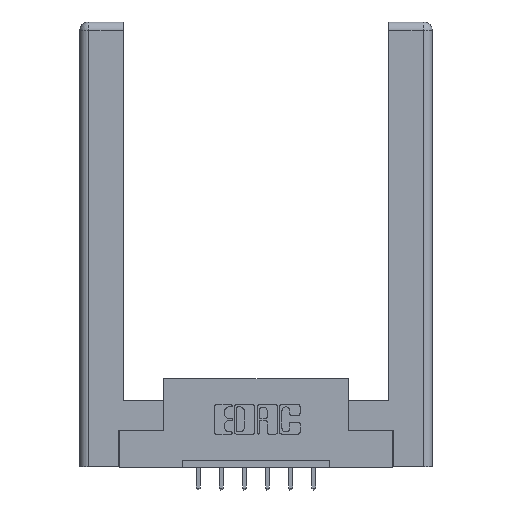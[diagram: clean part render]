
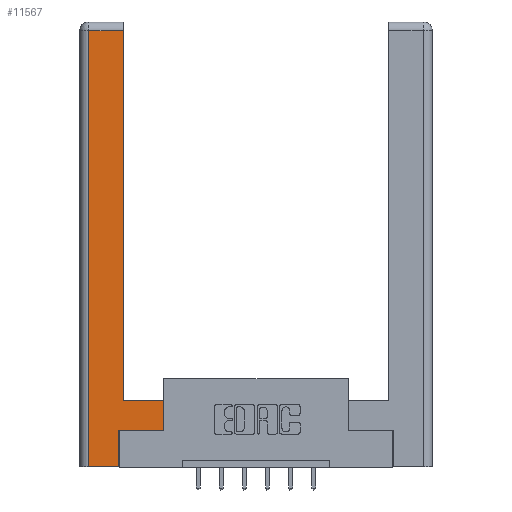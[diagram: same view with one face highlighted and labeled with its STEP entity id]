
A CAD part, top view. The second image highlights one B-rep face of the part: STEP entity #11567.
In plain terms, the highlighted planar face has unit normal (0, 0, 1).
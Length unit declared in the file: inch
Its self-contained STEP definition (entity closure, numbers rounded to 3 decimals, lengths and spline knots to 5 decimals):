
#91 = ORIENTED_EDGE ( 'NONE', *, *, #5771, .T. ) ;
#344 = CARTESIAN_POINT ( 'NONE',  ( 0.295, 3., 0. ) ) ;
#391 = CARTESIAN_POINT ( 'NONE',  ( 0.0615, 2.94, 0. ) ) ;
#846 = EDGE_CURVE ( 'NONE', #3905, #7077, #6645, .T. ) ;
#908 = ORIENTED_EDGE ( 'NONE', *, *, #11321, .T. ) ;
#1606 = CARTESIAN_POINT ( 'NONE',  ( 0.295, 2.94, 0. ) ) ;
#1679 = ORIENTED_EDGE ( 'NONE', *, *, #6896, .T. ) ;
#1963 = VERTEX_POINT ( 'NONE', #7099 ) ;
#2180 = LINE ( 'NONE', #7737, #3916 ) ;
#2184 = VERTEX_POINT ( 'NONE', #4002 ) ;
#2190 = VERTEX_POINT ( 'NONE', #3118 ) ;
#2525 = EDGE_CURVE ( 'NONE', #7077, #4217, #11561, .T. ) ;
#2612 = DIRECTION ( 'NONE',  ( -1., 0., 0. ) ) ;
#2654 = DIRECTION ( 'NONE',  ( 0., 0., -1. ) ) ;
#2847 = CARTESIAN_POINT ( 'NONE',  ( 0.265, 0.245, 0. ) ) ;
#3048 = DIRECTION ( 'NONE',  ( 0., 1., 0. ) ) ;
#3118 = CARTESIAN_POINT ( 'NONE',  ( 0.265, 0.245, 0. ) ) ;
#3319 = VERTEX_POINT ( 'NONE', #11004 ) ;
#3327 = VECTOR ( 'NONE', #5015, 39.37008 ) ;
#3403 = CARTESIAN_POINT ( 'NONE',  ( 0.0615, 2.94, 0. ) ) ;
#3614 = PLANE ( 'NONE',  #11242 ) ;
#3905 = VERTEX_POINT ( 'NONE', #5139 ) ;
#3916 = VECTOR ( 'NONE', #5990, 39.37008 ) ;
#3921 = ORIENTED_EDGE ( 'NONE', *, *, #846, .T. ) ;
#3953 = LINE ( 'NONE', #9154, #9455 ) ;
#4002 = CARTESIAN_POINT ( 'NONE',  ( 0.565, 0.45, 0. ) ) ;
#4118 = VERTEX_POINT ( 'NONE', #8397 ) ;
#4217 = VERTEX_POINT ( 'NONE', #391 ) ;
#4219 = LINE ( 'NONE', #4985, #10017 ) ;
#4470 = LINE ( 'NONE', #6733, #3327 ) ;
#4676 = DIRECTION ( 'NONE',  ( 0., -1., 0. ) ) ;
#4985 = CARTESIAN_POINT ( 'NONE',  ( 0.295, 0.45, 0. ) ) ;
#5015 = DIRECTION ( 'NONE',  ( 1., 0., 0. ) ) ;
#5139 = CARTESIAN_POINT ( 'NONE',  ( 0.295, 0.45, 0. ) ) ;
#5396 = DIRECTION ( 'NONE',  ( 0., 1., 0. ) ) ;
#5771 = EDGE_CURVE ( 'NONE', #4217, #3319, #3953, .T. ) ;
#5990 = DIRECTION ( 'NONE',  ( 0., 1., 0. ) ) ;
#6090 = DIRECTION ( 'NONE',  ( 1., 0., 0. ) ) ;
#6184 = FACE_OUTER_BOUND ( 'NONE', #6968, .T. ) ;
#6260 = CARTESIAN_POINT ( 'NONE',  ( 0., 0., 0. ) ) ;
#6645 = LINE ( 'NONE', #344, #9040 ) ;
#6733 = CARTESIAN_POINT ( 'NONE',  ( 0.265, 0., 0. ) ) ;
#6746 = ORIENTED_EDGE ( 'NONE', *, *, #8265, .T. ) ;
#6769 = ORIENTED_EDGE ( 'NONE', *, *, #7441, .T. ) ;
#6782 = ORIENTED_EDGE ( 'NONE', *, *, #7819, .T. ) ;
#6896 = EDGE_CURVE ( 'NONE', #1963, #2184, #2180, .T. ) ;
#6968 = EDGE_LOOP ( 'NONE', ( #3921, #9567, #91, #6769, #6782, #6746, #1679, #908 ) ) ;
#7077 = VERTEX_POINT ( 'NONE', #1606 ) ;
#7099 = CARTESIAN_POINT ( 'NONE',  ( 0.565, 0.245, 0. ) ) ;
#7441 = EDGE_CURVE ( 'NONE', #3319, #4118, #4470, .T. ) ;
#7737 = CARTESIAN_POINT ( 'NONE',  ( 0.565, 0.45, 0. ) ) ;
#7819 = EDGE_CURVE ( 'NONE', #4118, #2190, #8544, .T. ) ;
#8009 = VECTOR ( 'NONE', #10707, 39.37008 ) ;
#8265 = EDGE_CURVE ( 'NONE', #2190, #1963, #10802, .T. ) ;
#8390 = VECTOR ( 'NONE', #6090, 39.37008 ) ;
#8397 = CARTESIAN_POINT ( 'NONE',  ( 0.265, 0., 0. ) ) ;
#8544 = LINE ( 'NONE', #2847, #8680 ) ;
#8680 = VECTOR ( 'NONE', #5396, 39.37008 ) ;
#9040 = VECTOR ( 'NONE', #3048, 39.37008 ) ;
#9154 = CARTESIAN_POINT ( 'NONE',  ( 0.0615, 0., 0. ) ) ;
#9455 = VECTOR ( 'NONE', #4676, 39.37008 ) ;
#9567 = ORIENTED_EDGE ( 'NONE', *, *, #2525, .T. ) ;
#10017 = VECTOR ( 'NONE', #10420, 39.37008 ) ;
#10420 = DIRECTION ( 'NONE',  ( -1., 0., 0. ) ) ;
#10518 = CARTESIAN_POINT ( 'NONE',  ( 0.565, 0.245, 0. ) ) ;
#10707 = DIRECTION ( 'NONE',  ( -1., 0., 0. ) ) ;
#10802 = LINE ( 'NONE', #10518, #8390 ) ;
#11004 = CARTESIAN_POINT ( 'NONE',  ( 0.0615, 0., 0. ) ) ;
#11242 = AXIS2_PLACEMENT_3D ( 'NONE', #6260, #2654, #2612 ) ;
#11321 = EDGE_CURVE ( 'NONE', #2184, #3905, #4219, .T. ) ;
#11561 = LINE ( 'NONE', #3403, #8009 ) ;
#11567 = ADVANCED_FACE ( 'NONE', ( #6184 ), #3614, .F. ) ;
